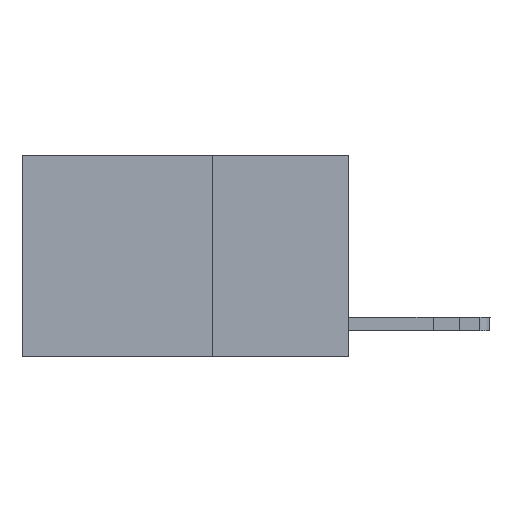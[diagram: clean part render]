
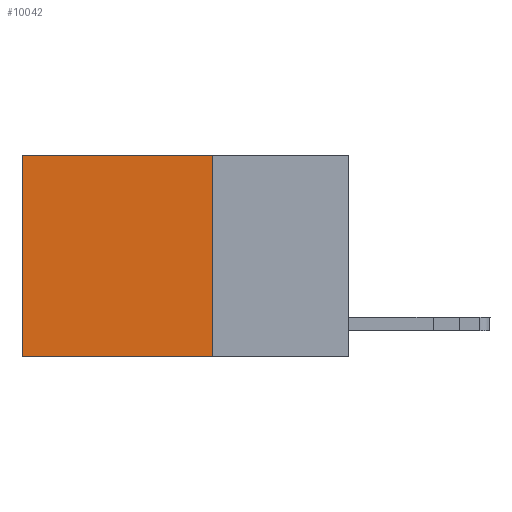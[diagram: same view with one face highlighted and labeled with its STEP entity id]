
A CAD part, left-side view. The second image highlights one B-rep face of the part: STEP entity #10042.
In plain terms, the highlighted planar face has unit normal (-1, 0, 0).
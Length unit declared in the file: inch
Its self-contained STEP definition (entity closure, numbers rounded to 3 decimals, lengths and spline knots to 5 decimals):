
#491 = EDGE_CURVE ( 'NONE', #2111, #9494, #6289, .T. ) ;
#1376 = EDGE_CURVE ( 'NONE', #7256, #1489, #15768, .T. ) ;
#1433 = EDGE_CURVE ( 'NONE', #9494, #1489, #1727, .T. ) ;
#1489 = VERTEX_POINT ( 'NONE', #8936 ) ;
#1727 = LINE ( 'NONE', #9750, #11540 ) ;
#1927 = DIRECTION ( 'NONE',  ( 0., 0., -1. ) ) ;
#2111 = VERTEX_POINT ( 'NONE', #2710 ) ;
#2710 = CARTESIAN_POINT ( 'NONE',  ( 0.2625, 0.25, 0. ) ) ;
#2841 = AXIS2_PLACEMENT_3D ( 'NONE', #4349, #6884, #15188 ) ;
#3536 = EDGE_LOOP ( 'NONE', ( #3584, #13824, #15248, #11491 ) ) ;
#3584 = ORIENTED_EDGE ( 'NONE', *, *, #1433, .T. ) ;
#4349 = CARTESIAN_POINT ( 'NONE',  ( 0.2625, 0.25, 0. ) ) ;
#4810 = DIRECTION ( 'NONE',  ( 0., 1., 0. ) ) ;
#5256 = LINE ( 'NONE', #9346, #8897 ) ;
#5863 = CARTESIAN_POINT ( 'NONE',  ( 0.2625, 0.6, 0. ) ) ;
#6289 = LINE ( 'NONE', #7829, #15423 ) ;
#6884 = DIRECTION ( 'NONE',  ( 1., 0., 0. ) ) ;
#6992 = EDGE_CURVE ( 'NONE', #2111, #7256, #5256, .T. ) ;
#7256 = VERTEX_POINT ( 'NONE', #9748 ) ;
#7829 = CARTESIAN_POINT ( 'NONE',  ( 0.2625, 0.25, 0. ) ) ;
#8443 = FACE_OUTER_BOUND ( 'NONE', #3536, .T. ) ;
#8743 = VECTOR ( 'NONE', #10312, 39.37008 ) ;
#8897 = VECTOR ( 'NONE', #1927, 39.37008 ) ;
#8936 = CARTESIAN_POINT ( 'NONE',  ( 0.2625, 0.6, -0.37 ) ) ;
#9346 = CARTESIAN_POINT ( 'NONE',  ( 0.2625, 0.25, 0. ) ) ;
#9494 = VERTEX_POINT ( 'NONE', #5863 ) ;
#9649 = DIRECTION ( 'NONE',  ( 0., 0., -1. ) ) ;
#9748 = CARTESIAN_POINT ( 'NONE',  ( 0.2625, 0.25, -0.37 ) ) ;
#9750 = CARTESIAN_POINT ( 'NONE',  ( 0.2625, 0.6, 0. ) ) ;
#10042 = ADVANCED_FACE ( 'NONE', ( #8443 ), #15138, .F. ) ;
#10312 = DIRECTION ( 'NONE',  ( 0., 1., 0. ) ) ;
#10400 = CARTESIAN_POINT ( 'NONE',  ( 0.2625, 0.25, -0.37 ) ) ;
#11491 = ORIENTED_EDGE ( 'NONE', *, *, #491, .T. ) ;
#11540 = VECTOR ( 'NONE', #9649, 39.37008 ) ;
#13824 = ORIENTED_EDGE ( 'NONE', *, *, #1376, .F. ) ;
#15138 = PLANE ( 'NONE',  #2841 ) ;
#15188 = DIRECTION ( 'NONE',  ( 0., 0., -1. ) ) ;
#15248 = ORIENTED_EDGE ( 'NONE', *, *, #6992, .F. ) ;
#15423 = VECTOR ( 'NONE', #4810, 39.37008 ) ;
#15768 = LINE ( 'NONE', #10400, #8743 ) ;
